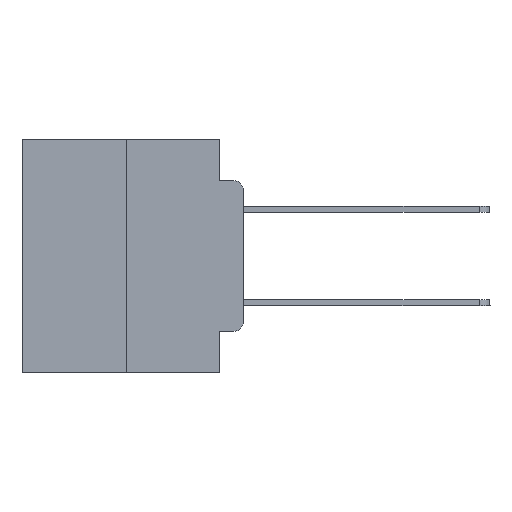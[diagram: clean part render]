
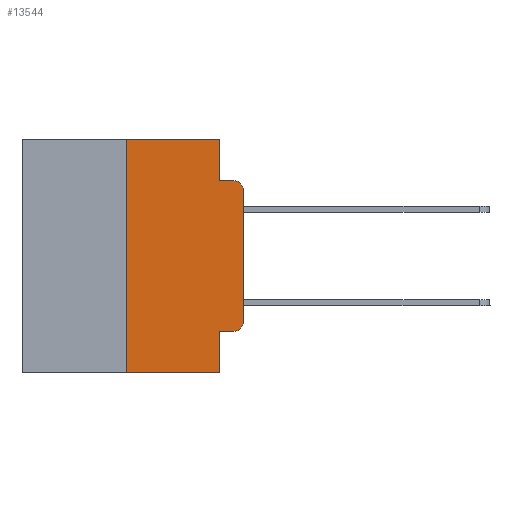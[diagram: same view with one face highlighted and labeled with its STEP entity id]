
A CAD part, left-side view. The second image highlights one B-rep face of the part: STEP entity #13544.
In plain terms, the highlighted planar face has unit normal (-1, 0, 0).
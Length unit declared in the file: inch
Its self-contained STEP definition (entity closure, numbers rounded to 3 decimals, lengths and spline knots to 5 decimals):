
#122 = CARTESIAN_POINT ( 'NONE',  ( 0., 0.051, 0. ) ) ;
#547 = EDGE_CURVE ( 'NONE', #23724, #15707, #1417, .T. ) ;
#1417 = CIRCLE ( 'NONE', #17139, 0.02 ) ;
#1601 = VECTOR ( 'NONE', #16386, 39.37008 ) ;
#1674 = LINE ( 'NONE', #5782, #25487 ) ;
#2066 = DIRECTION ( 'NONE',  ( 1., 0., 0. ) ) ;
#2121 = LINE ( 'NONE', #8463, #16863 ) ;
#2425 = ORIENTED_EDGE ( 'NONE', *, *, #19339, .F. ) ;
#2968 = CARTESIAN_POINT ( 'NONE',  ( 0., 0.25, -0.5 ) ) ;
#3230 = DIRECTION ( 'NONE',  ( 0., 0., -1. ) ) ;
#3299 = DIRECTION ( 'NONE',  ( 0., -1., 0. ) ) ;
#3365 = CARTESIAN_POINT ( 'NONE',  ( 0., 0.051, 0. ) ) ;
#3671 = DIRECTION ( 'NONE',  ( 0., -1., 0. ) ) ;
#3978 = VECTOR ( 'NONE', #3299, 39.37008 ) ;
#4028 = DIRECTION ( 'NONE',  ( 0., 0., -1. ) ) ;
#4474 = CARTESIAN_POINT ( 'NONE',  ( 0., 0.051, 0. ) ) ;
#4916 = CARTESIAN_POINT ( 'NONE',  ( 0., 0.02, -0.0885 ) ) ;
#5607 = CARTESIAN_POINT ( 'NONE',  ( 0., 0.051, -0.4115 ) ) ;
#5782 = CARTESIAN_POINT ( 'NONE',  ( 0., 0.473, 0. ) ) ;
#6363 = DIRECTION ( 'NONE',  ( 0., 0., 1. ) ) ;
#6415 = ORIENTED_EDGE ( 'NONE', *, *, #20043, .F. ) ;
#6576 = CARTESIAN_POINT ( 'NONE',  ( 0., 0.25, 0. ) ) ;
#6862 = PLANE ( 'NONE',  #17612 ) ;
#6965 = CARTESIAN_POINT ( 'NONE',  ( 0., 0.473, -0.5 ) ) ;
#7031 = VERTEX_POINT ( 'NONE', #22027 ) ;
#7937 = LINE ( 'NONE', #27210, #3978 ) ;
#8089 = VERTEX_POINT ( 'NONE', #5607 ) ;
#8095 = CARTESIAN_POINT ( 'NONE',  ( 0., 0.051, -0.0885 ) ) ;
#8390 = CARTESIAN_POINT ( 'NONE',  ( 0., 0., 0. ) ) ;
#8463 = CARTESIAN_POINT ( 'NONE',  ( 0., 0.25, 0. ) ) ;
#8727 = VECTOR ( 'NONE', #16964, 39.37008 ) ;
#8969 = DIRECTION ( 'NONE',  ( 0., 0., -1. ) ) ;
#8985 = LINE ( 'NONE', #4474, #22356 ) ;
#9359 = VERTEX_POINT ( 'NONE', #2968 ) ;
#10220 = ORIENTED_EDGE ( 'NONE', *, *, #24034, .T. ) ;
#10592 = DIRECTION ( 'NONE',  ( 0., 0., -1. ) ) ;
#11998 = VERTEX_POINT ( 'NONE', #23068 ) ;
#12153 = VERTEX_POINT ( 'NONE', #6576 ) ;
#12232 = VERTEX_POINT ( 'NONE', #27548 ) ;
#12460 = CARTESIAN_POINT ( 'NONE',  ( 0., 0.02, -0.1085 ) ) ;
#12968 = VECTOR ( 'NONE', #20188, 39.37008 ) ;
#13026 = LINE ( 'NONE', #8390, #8727 ) ;
#13544 = ADVANCED_FACE ( 'NONE', ( #21491 ), #6862, .F. ) ;
#14185 = ORIENTED_EDGE ( 'NONE', *, *, #23158, .F. ) ;
#14878 = DIRECTION ( 'NONE',  ( 0., 0., -1. ) ) ;
#15212 = CARTESIAN_POINT ( 'NONE',  ( 0., 0.02, -0.3915 ) ) ;
#15344 = VERTEX_POINT ( 'NONE', #27432 ) ;
#15707 = VERTEX_POINT ( 'NONE', #4916 ) ;
#15967 = ORIENTED_EDGE ( 'NONE', *, *, #547, .T. ) ;
#16064 = EDGE_CURVE ( 'NONE', #15344, #23724, #13026, .T. ) ;
#16386 = DIRECTION ( 'NONE',  ( 0., -1., 0. ) ) ;
#16517 = LINE ( 'NONE', #8095, #1601 ) ;
#16863 = VECTOR ( 'NONE', #6363, 39.37008 ) ;
#16964 = DIRECTION ( 'NONE',  ( 0., 0., 1. ) ) ;
#17139 = AXIS2_PLACEMENT_3D ( 'NONE', #12460, #25167, #4028 ) ;
#17193 = DIRECTION ( 'NONE',  ( -1., 0., 0. ) ) ;
#17612 = AXIS2_PLACEMENT_3D ( 'NONE', #23759, #2066, #14878 ) ;
#19217 = AXIS2_PLACEMENT_3D ( 'NONE', #15212, #17193, #10592 ) ;
#19339 = EDGE_CURVE ( 'NONE', #9359, #12153, #2121, .T. ) ;
#20043 = EDGE_CURVE ( 'NONE', #7031, #15707, #16517, .T. ) ;
#20084 = ORIENTED_EDGE ( 'NONE', *, *, #20979, .F. ) ;
#20188 = DIRECTION ( 'NONE',  ( 0., -1., 0. ) ) ;
#20530 = LINE ( 'NONE', #3365, #25523 ) ;
#20567 = CIRCLE ( 'NONE', #19217, 0.02 ) ;
#20613 = ORIENTED_EDGE ( 'NONE', *, *, #23370, .F. ) ;
#20979 = EDGE_CURVE ( 'NONE', #12153, #27139, #1674, .T. ) ;
#21491 = FACE_OUTER_BOUND ( 'NONE', #21834, .T. ) ;
#21834 = EDGE_LOOP ( 'NONE', ( #26633, #15967, #6415, #20613, #20084, #2425, #22650, #14185, #10220, #25174 ) ) ;
#22027 = CARTESIAN_POINT ( 'NONE',  ( 0., 0.051, -0.0885 ) ) ;
#22048 = EDGE_CURVE ( 'NONE', #11998, #15344, #20567, .T. ) ;
#22356 = VECTOR ( 'NONE', #8969, 39.37008 ) ;
#22650 = ORIENTED_EDGE ( 'NONE', *, *, #24004, .T. ) ;
#22747 = CARTESIAN_POINT ( 'NONE',  ( 0., 0., -0.1085 ) ) ;
#23068 = CARTESIAN_POINT ( 'NONE',  ( 0., 0.02, -0.4115 ) ) ;
#23158 = EDGE_CURVE ( 'NONE', #8089, #12232, #20530, .T. ) ;
#23370 = EDGE_CURVE ( 'NONE', #27139, #7031, #8985, .T. ) ;
#23724 = VERTEX_POINT ( 'NONE', #22747 ) ;
#23759 = CARTESIAN_POINT ( 'NONE',  ( 0., 0.473, 0. ) ) ;
#24004 = EDGE_CURVE ( 'NONE', #9359, #12232, #26250, .T. ) ;
#24034 = EDGE_CURVE ( 'NONE', #8089, #11998, #7937, .T. ) ;
#25167 = DIRECTION ( 'NONE',  ( -1., 0., 0. ) ) ;
#25174 = ORIENTED_EDGE ( 'NONE', *, *, #22048, .T. ) ;
#25487 = VECTOR ( 'NONE', #3671, 39.37008 ) ;
#25523 = VECTOR ( 'NONE', #3230, 39.37008 ) ;
#26250 = LINE ( 'NONE', #6965, #12968 ) ;
#26633 = ORIENTED_EDGE ( 'NONE', *, *, #16064, .T. ) ;
#27139 = VERTEX_POINT ( 'NONE', #122 ) ;
#27210 = CARTESIAN_POINT ( 'NONE',  ( 0., 0.051, -0.4115 ) ) ;
#27432 = CARTESIAN_POINT ( 'NONE',  ( 0., 0., -0.3915 ) ) ;
#27548 = CARTESIAN_POINT ( 'NONE',  ( 0., 0.051, -0.5 ) ) ;
